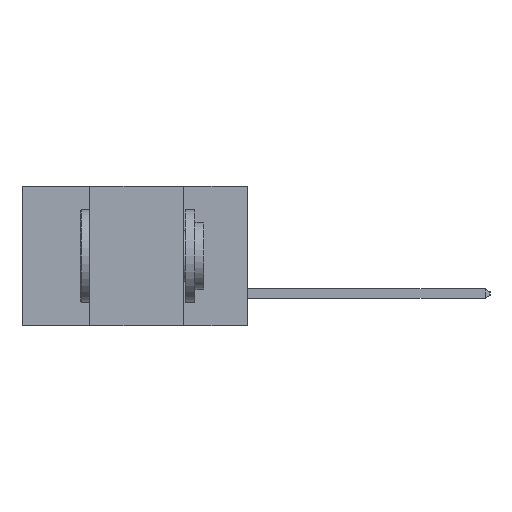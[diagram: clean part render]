
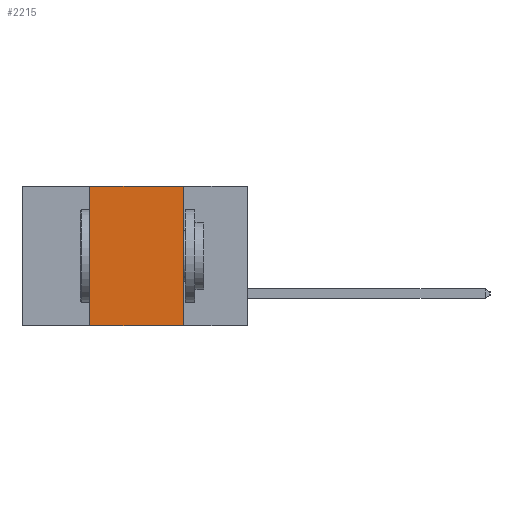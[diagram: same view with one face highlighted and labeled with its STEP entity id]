
A CAD part, left-side view. The second image highlights one B-rep face of the part: STEP entity #2215.
In plain terms, the highlighted planar face has unit normal (-1, 0, 0).
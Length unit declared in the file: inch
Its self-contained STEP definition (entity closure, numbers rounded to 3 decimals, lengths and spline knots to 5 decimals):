
#973 = CARTESIAN_POINT ( 'NONE',  ( 0., 0.42, -0.37 ) ) ;
#1180 = EDGE_LOOP ( 'NONE', ( #13435, #4312, #11986, #11500 ) ) ;
#2215 = ADVANCED_FACE ( 'NONE', ( #13058 ), #17396, .F. ) ;
#2450 = CARTESIAN_POINT ( 'NONE',  ( 0., 0.42, -0.37 ) ) ;
#2889 = DIRECTION ( 'NONE',  ( 0., 0., -1. ) ) ;
#3209 = LINE ( 'NONE', #9934, #14924 ) ;
#4033 = DIRECTION ( 'NONE',  ( 0., 0., 1. ) ) ;
#4312 = ORIENTED_EDGE ( 'NONE', *, *, #5111, .F. ) ;
#4885 = DIRECTION ( 'NONE',  ( 0., -1., 0. ) ) ;
#5086 = CARTESIAN_POINT ( 'NONE',  ( 0., 0.6, 0. ) ) ;
#5111 = EDGE_CURVE ( 'NONE', #12534, #12737, #5940, .T. ) ;
#5243 = CARTESIAN_POINT ( 'NONE',  ( 0., 0.17, -0.37 ) ) ;
#5752 = AXIS2_PLACEMENT_3D ( 'NONE', #17195, #17090, #17067 ) ;
#5940 = LINE ( 'NONE', #5086, #13654 ) ;
#6847 = VECTOR ( 'NONE', #2889, 39.37008 ) ;
#7418 = CARTESIAN_POINT ( 'NONE',  ( 0., 0.17, -0.37 ) ) ;
#9934 = CARTESIAN_POINT ( 'NONE',  ( 0., 0.6, -0.37 ) ) ;
#10614 = CARTESIAN_POINT ( 'NONE',  ( 0., 0.42, 0. ) ) ;
#11494 = LINE ( 'NONE', #7418, #6847 ) ;
#11500 = ORIENTED_EDGE ( 'NONE', *, *, #19222, .T. ) ;
#11527 = DIRECTION ( 'NONE',  ( 0., -1., 0. ) ) ;
#11562 = VECTOR ( 'NONE', #4033, 39.37008 ) ;
#11986 = ORIENTED_EDGE ( 'NONE', *, *, #12979, .F. ) ;
#12534 = VERTEX_POINT ( 'NONE', #10614 ) ;
#12737 = VERTEX_POINT ( 'NONE', #15676 ) ;
#12979 = EDGE_CURVE ( 'NONE', #16020, #12534, #19494, .T. ) ;
#13058 = FACE_OUTER_BOUND ( 'NONE', #1180, .T. ) ;
#13435 = ORIENTED_EDGE ( 'NONE', *, *, #16128, .F. ) ;
#13654 = VECTOR ( 'NONE', #4885, 39.37008 ) ;
#14924 = VECTOR ( 'NONE', #11527, 39.37008 ) ;
#15676 = CARTESIAN_POINT ( 'NONE',  ( 0., 0.17, 0. ) ) ;
#16020 = VERTEX_POINT ( 'NONE', #973 ) ;
#16128 = EDGE_CURVE ( 'NONE', #12737, #19018, #11494, .T. ) ;
#17067 = DIRECTION ( 'NONE',  ( 0., 0., -1. ) ) ;
#17090 = DIRECTION ( 'NONE',  ( 1., 0., 0. ) ) ;
#17195 = CARTESIAN_POINT ( 'NONE',  ( 0., 0.6, 0. ) ) ;
#17396 = PLANE ( 'NONE',  #5752 ) ;
#19018 = VERTEX_POINT ( 'NONE', #5243 ) ;
#19222 = EDGE_CURVE ( 'NONE', #16020, #19018, #3209, .T. ) ;
#19494 = LINE ( 'NONE', #2450, #11562 ) ;
